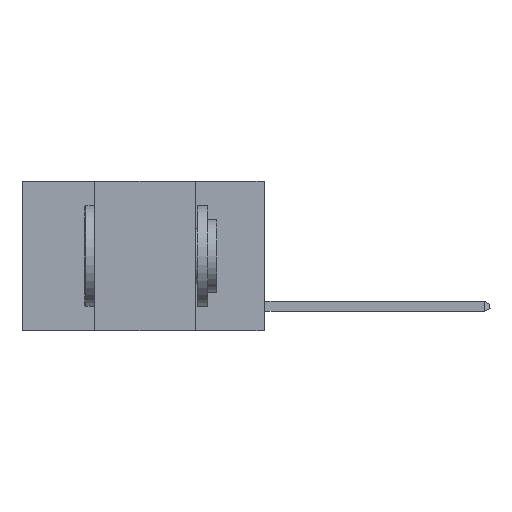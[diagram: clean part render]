
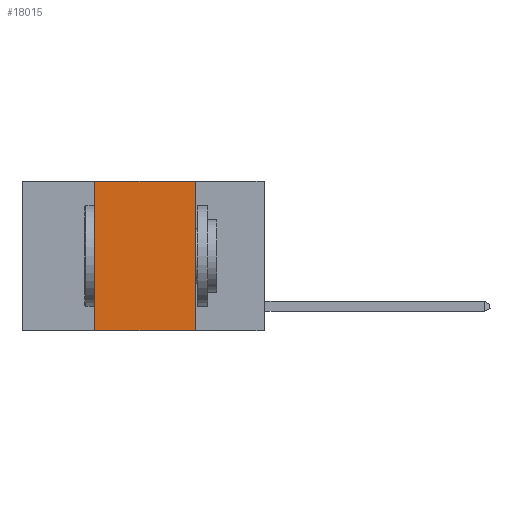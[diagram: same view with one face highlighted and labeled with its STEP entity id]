
A CAD part, left-side view. The second image highlights one B-rep face of the part: STEP entity #18015.
In plain terms, the highlighted planar face has unit normal (-1, 0, 0).
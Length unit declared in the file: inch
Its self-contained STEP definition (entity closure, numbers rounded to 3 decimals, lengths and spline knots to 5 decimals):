
#1009 = DIRECTION ( 'NONE',  ( 0., 0., -1. ) ) ;
#1294 = CARTESIAN_POINT ( 'NONE',  ( 0., 0.17, 0. ) ) ;
#2042 = AXIS2_PLACEMENT_3D ( 'NONE', #9468, #10910, #2488 ) ;
#2488 = DIRECTION ( 'NONE',  ( 0., 0., -1. ) ) ;
#3636 = EDGE_CURVE ( 'NONE', #4680, #11652, #5388, .T. ) ;
#4680 = VERTEX_POINT ( 'NONE', #15380 ) ;
#5305 = FACE_OUTER_BOUND ( 'NONE', #9134, .T. ) ;
#5388 = LINE ( 'NONE', #1294, #8651 ) ;
#5639 = CARTESIAN_POINT ( 'NONE',  ( 0., 0.42, 0. ) ) ;
#5651 = VECTOR ( 'NONE', #5768, 39.37008 ) ;
#5768 = DIRECTION ( 'NONE',  ( 0., -1., 0. ) ) ;
#6530 = VECTOR ( 'NONE', #15361, 39.37008 ) ;
#7364 = DIRECTION ( 'NONE',  ( 0., -1., 0. ) ) ;
#7881 = ORIENTED_EDGE ( 'NONE', *, *, #3636, .F. ) ;
#8079 = PLANE ( 'NONE',  #2042 ) ;
#8651 = VECTOR ( 'NONE', #1009, 39.37008 ) ;
#9032 = EDGE_CURVE ( 'NONE', #13347, #11652, #17520, .T. ) ;
#9134 = EDGE_LOOP ( 'NONE', ( #7881, #14630, #10061, #10953 ) ) ;
#9345 = LINE ( 'NONE', #11327, #5651 ) ;
#9468 = CARTESIAN_POINT ( 'NONE',  ( 0., 0.6, 0. ) ) ;
#9769 = CARTESIAN_POINT ( 'NONE',  ( 0., 0.42, 0. ) ) ;
#10061 = ORIENTED_EDGE ( 'NONE', *, *, #14789, .F. ) ;
#10910 = DIRECTION ( 'NONE',  ( 1., 0., 0. ) ) ;
#10953 = ORIENTED_EDGE ( 'NONE', *, *, #9032, .T. ) ;
#11327 = CARTESIAN_POINT ( 'NONE',  ( 0., 0.6, 0. ) ) ;
#11652 = VERTEX_POINT ( 'NONE', #13424 ) ;
#11710 = CARTESIAN_POINT ( 'NONE',  ( 0., 0.6, -0.37 ) ) ;
#12335 = CARTESIAN_POINT ( 'NONE',  ( 0., 0.42, -0.37 ) ) ;
#12946 = VERTEX_POINT ( 'NONE', #9769 ) ;
#13347 = VERTEX_POINT ( 'NONE', #12335 ) ;
#13424 = CARTESIAN_POINT ( 'NONE',  ( 0., 0.17, -0.37 ) ) ;
#14630 = ORIENTED_EDGE ( 'NONE', *, *, #14823, .F. ) ;
#14789 = EDGE_CURVE ( 'NONE', #13347, #12946, #17619, .T. ) ;
#14823 = EDGE_CURVE ( 'NONE', #12946, #4680, #9345, .T. ) ;
#15361 = DIRECTION ( 'NONE',  ( 0., 0., 1. ) ) ;
#15380 = CARTESIAN_POINT ( 'NONE',  ( 0., 0.17, 0. ) ) ;
#16674 = VECTOR ( 'NONE', #7364, 39.37008 ) ;
#17520 = LINE ( 'NONE', #11710, #16674 ) ;
#17619 = LINE ( 'NONE', #5639, #6530 ) ;
#18015 = ADVANCED_FACE ( 'NONE', ( #5305 ), #8079, .F. ) ;
